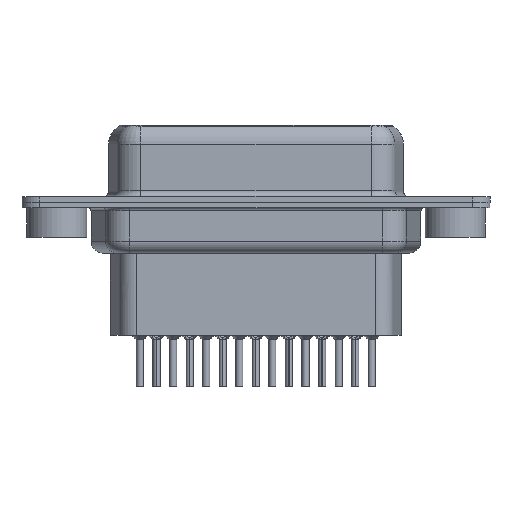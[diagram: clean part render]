
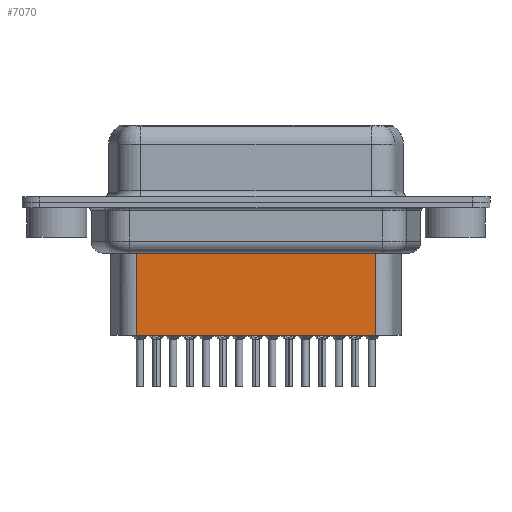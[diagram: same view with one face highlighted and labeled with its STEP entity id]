
A CAD part, front view. The second image highlights one B-rep face of the part: STEP entity #7070.
In plain terms, the highlighted planar face has unit normal (0, -1, 0).
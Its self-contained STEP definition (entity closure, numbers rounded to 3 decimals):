
#500 = EDGE_LOOP ( 'NONE', ( #15112, #5912, #3490, #10260 ) ) ;
#2045 = CARTESIAN_POINT ( 'NONE',  ( 6.681, -3.5, -11.15 ) ) ;
#3406 = VERTEX_POINT ( 'NONE', #23179 ) ;
#3490 = ORIENTED_EDGE ( 'NONE', *, *, #7935, .T. ) ;
#3861 = DIRECTION ( 'NONE',  ( -1., 0., 0. ) ) ;
#3978 = LINE ( 'NONE', #2045, #8052 ) ;
#4032 = EDGE_CURVE ( 'NONE', #21926, #13570, #9557, .T. ) ;
#5024 = DIRECTION ( 'NONE',  ( 1., 0., 0. ) ) ;
#5490 = VERTEX_POINT ( 'NONE', #18135 ) ;
#5912 = ORIENTED_EDGE ( 'NONE', *, *, #11079, .T. ) ;
#6220 = VECTOR ( 'NONE', #20204, 1000. ) ;
#6629 = CARTESIAN_POINT ( 'NONE',  ( 6.434, -3.5, -4.097 ) ) ;
#6838 = PLANE ( 'NONE',  #23429 ) ;
#7070 = ADVANCED_FACE ( 'NONE', ( #23454 ), #6838, .T. ) ;
#7935 = EDGE_CURVE ( 'NONE', #5490, #3406, #22369, .T. ) ;
#8052 = VECTOR ( 'NONE', #3861, 1000. ) ;
#8441 = LINE ( 'NONE', #6629, #6220 ) ;
#9557 = LINE ( 'NONE', #16911, #13571 ) ;
#10260 = ORIENTED_EDGE ( 'NONE', *, *, #22947, .F. ) ;
#11079 = EDGE_CURVE ( 'NONE', #21926, #5490, #8441, .T. ) ;
#11486 = DIRECTION ( 'NONE',  ( 0., 0., -1. ) ) ;
#12220 = VECTOR ( 'NONE', #13135, 1000. ) ;
#13135 = DIRECTION ( 'NONE',  ( 0., 0., -1. ) ) ;
#13570 = VERTEX_POINT ( 'NONE', #19385 ) ;
#13571 = VECTOR ( 'NONE', #11486, 1000. ) ;
#14206 = CARTESIAN_POINT ( 'NONE',  ( 6.681, -3.5, -3.1 ) ) ;
#14322 = DIRECTION ( 'NONE',  ( 0., -1., 0. ) ) ;
#15112 = ORIENTED_EDGE ( 'NONE', *, *, #4032, .F. ) ;
#16911 = CARTESIAN_POINT ( 'NONE',  ( 26.619, -3.5, -3.1 ) ) ;
#17117 = CARTESIAN_POINT ( 'NONE',  ( 6.681, -3.5, -3.1 ) ) ;
#17717 = CARTESIAN_POINT ( 'NONE',  ( 26.619, -3.5, -4.097 ) ) ;
#18135 = CARTESIAN_POINT ( 'NONE',  ( 6.681, -3.5, -4.097 ) ) ;
#19385 = CARTESIAN_POINT ( 'NONE',  ( 26.619, -3.5, -11.15 ) ) ;
#20204 = DIRECTION ( 'NONE',  ( -1., 0., 0. ) ) ;
#21926 = VERTEX_POINT ( 'NONE', #17717 ) ;
#22369 = LINE ( 'NONE', #17117, #12220 ) ;
#22947 = EDGE_CURVE ( 'NONE', #13570, #3406, #3978, .T. ) ;
#23179 = CARTESIAN_POINT ( 'NONE',  ( 6.681, -3.5, -11.15 ) ) ;
#23429 = AXIS2_PLACEMENT_3D ( 'NONE', #14206, #14322, #5024 ) ;
#23454 = FACE_OUTER_BOUND ( 'NONE', #500, .T. ) ;
